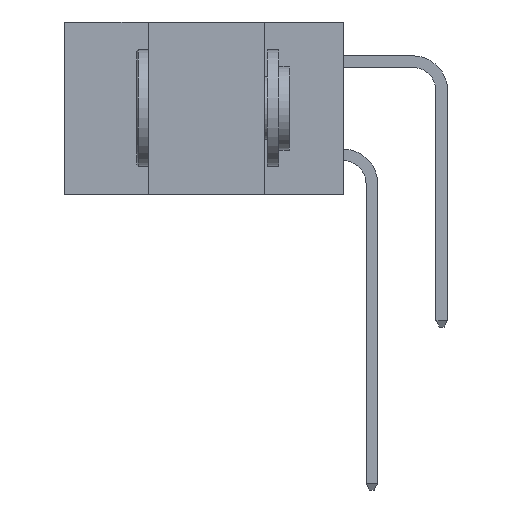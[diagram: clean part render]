
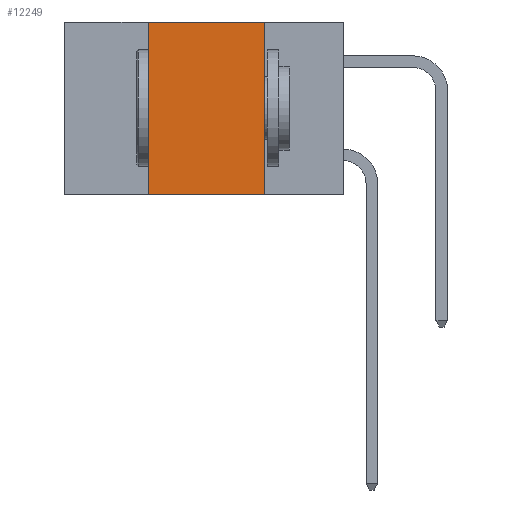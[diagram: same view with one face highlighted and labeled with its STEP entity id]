
A CAD part, left-side view. The second image highlights one B-rep face of the part: STEP entity #12249.
In plain terms, the highlighted planar face has unit normal (-1, 0, 0).
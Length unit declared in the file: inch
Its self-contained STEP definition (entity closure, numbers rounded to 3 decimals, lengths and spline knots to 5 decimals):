
#827 = EDGE_LOOP ( 'NONE', ( #9533, #4367, #12596, #10880 ) ) ;
#2117 = LINE ( 'NONE', #3175, #8992 ) ;
#2444 = DIRECTION ( 'NONE',  ( 0., -1., 0. ) ) ;
#2772 = EDGE_CURVE ( 'NONE', #10067, #9032, #16188, .T. ) ;
#2977 = DIRECTION ( 'NONE',  ( 0., 0., 1. ) ) ;
#3025 = CARTESIAN_POINT ( 'NONE',  ( 0., 0.6, -0.37 ) ) ;
#3175 = CARTESIAN_POINT ( 'NONE',  ( 0., 0.42, -0.37 ) ) ;
#3657 = DIRECTION ( 'NONE',  ( 0., 0., -1. ) ) ;
#3713 = CARTESIAN_POINT ( 'NONE',  ( 0., 0.17, -0.37 ) ) ;
#4367 = ORIENTED_EDGE ( 'NONE', *, *, #2772, .F. ) ;
#4521 = VERTEX_POINT ( 'NONE', #9768 ) ;
#4952 = CARTESIAN_POINT ( 'NONE',  ( 0., 0.17, 0. ) ) ;
#5064 = LINE ( 'NONE', #3025, #5431 ) ;
#5431 = VECTOR ( 'NONE', #14244, 39.37008 ) ;
#5689 = VERTEX_POINT ( 'NONE', #11482 ) ;
#5870 = AXIS2_PLACEMENT_3D ( 'NONE', #15035, #16213, #9007 ) ;
#6462 = VECTOR ( 'NONE', #2444, 39.37008 ) ;
#6464 = PLANE ( 'NONE',  #5870 ) ;
#7683 = EDGE_CURVE ( 'NONE', #9032, #5689, #9577, .T. ) ;
#8003 = EDGE_CURVE ( 'NONE', #4521, #10067, #2117, .T. ) ;
#8992 = VECTOR ( 'NONE', #2977, 39.37008 ) ;
#9007 = DIRECTION ( 'NONE',  ( 0., 0., -1. ) ) ;
#9032 = VERTEX_POINT ( 'NONE', #4952 ) ;
#9533 = ORIENTED_EDGE ( 'NONE', *, *, #7683, .F. ) ;
#9577 = LINE ( 'NONE', #3713, #15982 ) ;
#9768 = CARTESIAN_POINT ( 'NONE',  ( 0., 0.42, -0.37 ) ) ;
#10067 = VERTEX_POINT ( 'NONE', #15478 ) ;
#10880 = ORIENTED_EDGE ( 'NONE', *, *, #13206, .T. ) ;
#11482 = CARTESIAN_POINT ( 'NONE',  ( 0., 0.17, -0.37 ) ) ;
#12249 = ADVANCED_FACE ( 'NONE', ( #16029 ), #6464, .F. ) ;
#12596 = ORIENTED_EDGE ( 'NONE', *, *, #8003, .F. ) ;
#13206 = EDGE_CURVE ( 'NONE', #4521, #5689, #5064, .T. ) ;
#14244 = DIRECTION ( 'NONE',  ( 0., -1., 0. ) ) ;
#14403 = CARTESIAN_POINT ( 'NONE',  ( 0., 0.6, 0. ) ) ;
#15035 = CARTESIAN_POINT ( 'NONE',  ( 0., 0.6, 0. ) ) ;
#15478 = CARTESIAN_POINT ( 'NONE',  ( 0., 0.42, 0. ) ) ;
#15982 = VECTOR ( 'NONE', #3657, 39.37008 ) ;
#16029 = FACE_OUTER_BOUND ( 'NONE', #827, .T. ) ;
#16188 = LINE ( 'NONE', #14403, #6462 ) ;
#16213 = DIRECTION ( 'NONE',  ( 1., 0., 0. ) ) ;
